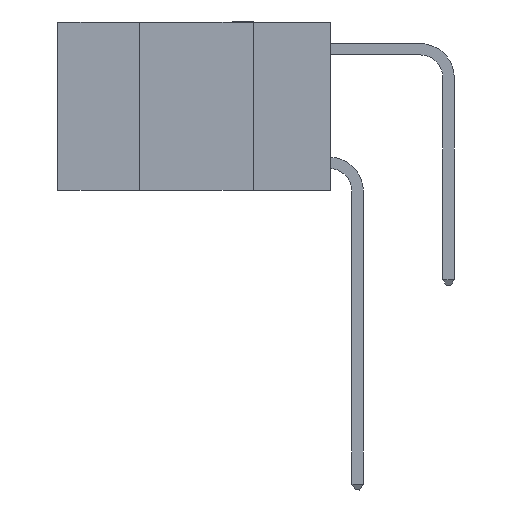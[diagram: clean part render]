
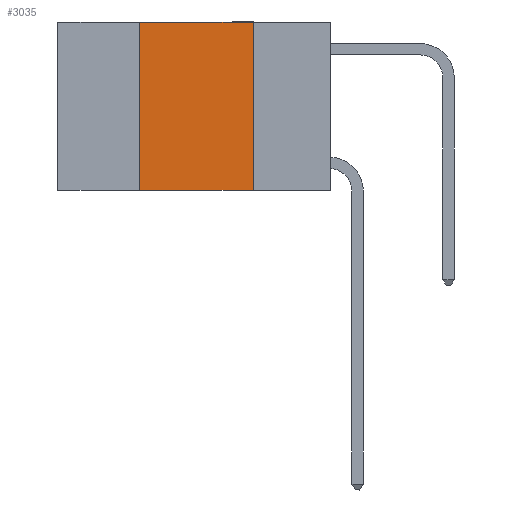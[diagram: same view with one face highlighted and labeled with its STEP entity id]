
A CAD part, left-side view. The second image highlights one B-rep face of the part: STEP entity #3035.
In plain terms, the highlighted planar face has unit normal (-1, 0, 0).
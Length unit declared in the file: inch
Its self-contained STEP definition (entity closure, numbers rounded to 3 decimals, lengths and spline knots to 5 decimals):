
#434 = FACE_OUTER_BOUND ( 'NONE', #9174, .T. ) ;
#458 = CARTESIAN_POINT ( 'NONE',  ( 0., 0.17, 0. ) ) ;
#645 = CARTESIAN_POINT ( 'NONE',  ( 0., 0.6, 0. ) ) ;
#812 = DIRECTION ( 'NONE',  ( 0., -1., 0. ) ) ;
#821 = VERTEX_POINT ( 'NONE', #458 ) ;
#852 = DIRECTION ( 'NONE',  ( 0., 0., -1. ) ) ;
#864 = DIRECTION ( 'NONE',  ( 1., 0., 0. ) ) ;
#906 = CARTESIAN_POINT ( 'NONE',  ( 0., 0.6, 0. ) ) ;
#936 = PLANE ( 'NONE',  #3338 ) ;
#1737 = LINE ( 'NONE', #7046, #12155 ) ;
#1888 = CARTESIAN_POINT ( 'NONE',  ( 0., 0.42, -0.37 ) ) ;
#2492 = EDGE_CURVE ( 'NONE', #11251, #5813, #8678, .T. ) ;
#3035 = ADVANCED_FACE ( 'NONE', ( #434 ), #936, .F. ) ;
#3062 = EDGE_CURVE ( 'NONE', #12574, #821, #10966, .T. ) ;
#3338 = AXIS2_PLACEMENT_3D ( 'NONE', #906, #864, #852 ) ;
#5009 = CARTESIAN_POINT ( 'NONE',  ( 0., 0.17, 0. ) ) ;
#5368 = VECTOR ( 'NONE', #812, 39.37008 ) ;
#5524 = LINE ( 'NONE', #5009, #13449 ) ;
#5813 = VERTEX_POINT ( 'NONE', #8600 ) ;
#6069 = DIRECTION ( 'NONE',  ( 0., 0., -1. ) ) ;
#7046 = CARTESIAN_POINT ( 'NONE',  ( 0., 0.42, 0. ) ) ;
#8412 = EDGE_CURVE ( 'NONE', #821, #5813, #5524, .T. ) ;
#8600 = CARTESIAN_POINT ( 'NONE',  ( 0., 0.17, -0.37 ) ) ;
#8678 = LINE ( 'NONE', #8875, #11148 ) ;
#8797 = DIRECTION ( 'NONE',  ( 0., -1., 0. ) ) ;
#8875 = CARTESIAN_POINT ( 'NONE',  ( 0., 0.6, -0.37 ) ) ;
#9174 = EDGE_LOOP ( 'NONE', ( #11420, #11583, #12014, #12076 ) ) ;
#10351 = CARTESIAN_POINT ( 'NONE',  ( 0., 0.42, 0. ) ) ;
#10966 = LINE ( 'NONE', #645, #5368 ) ;
#11148 = VECTOR ( 'NONE', #8797, 39.37008 ) ;
#11251 = VERTEX_POINT ( 'NONE', #1888 ) ;
#11420 = ORIENTED_EDGE ( 'NONE', *, *, #8412, .F. ) ;
#11583 = ORIENTED_EDGE ( 'NONE', *, *, #3062, .F. ) ;
#12014 = ORIENTED_EDGE ( 'NONE', *, *, #12473, .F. ) ;
#12076 = ORIENTED_EDGE ( 'NONE', *, *, #2492, .T. ) ;
#12155 = VECTOR ( 'NONE', #12276, 39.37008 ) ;
#12276 = DIRECTION ( 'NONE',  ( 0., 0., 1. ) ) ;
#12473 = EDGE_CURVE ( 'NONE', #11251, #12574, #1737, .T. ) ;
#12574 = VERTEX_POINT ( 'NONE', #10351 ) ;
#13449 = VECTOR ( 'NONE', #6069, 39.37008 ) ;
